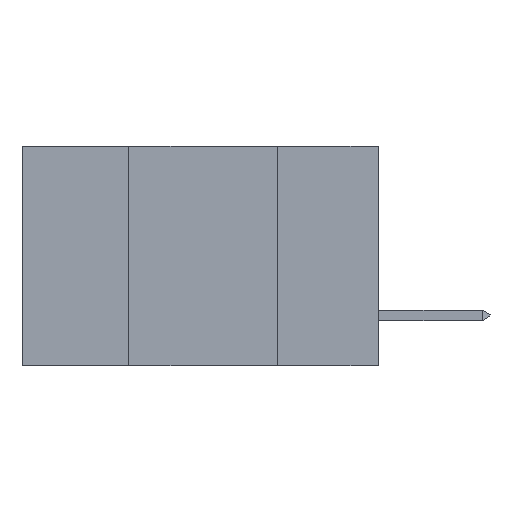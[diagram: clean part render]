
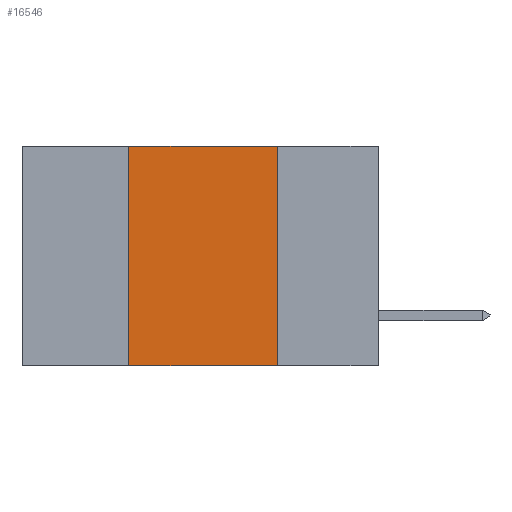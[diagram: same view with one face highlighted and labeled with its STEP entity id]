
A CAD part, left-side view. The second image highlights one B-rep face of the part: STEP entity #16546.
In plain terms, the highlighted planar face has unit normal (-1, 0, 0).
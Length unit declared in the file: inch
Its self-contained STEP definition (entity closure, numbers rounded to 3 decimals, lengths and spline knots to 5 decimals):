
#92 = CARTESIAN_POINT ( 'NONE',  ( 0., 0.42, -0.37 ) ) ;
#449 = DIRECTION ( 'NONE',  ( 0., -1., 0. ) ) ;
#776 = DIRECTION ( 'NONE',  ( 0., 0., -1. ) ) ;
#977 = CARTESIAN_POINT ( 'NONE',  ( 0., 0.17, -0.37 ) ) ;
#1224 = DIRECTION ( 'NONE',  ( 0., -1., 0. ) ) ;
#1528 = VERTEX_POINT ( 'NONE', #7493 ) ;
#1850 = VECTOR ( 'NONE', #1224, 39.37008 ) ;
#1912 = LINE ( 'NONE', #7753, #3052 ) ;
#3052 = VECTOR ( 'NONE', #449, 39.37008 ) ;
#4154 = DIRECTION ( 'NONE',  ( 0., 0., -1. ) ) ;
#5501 = PLANE ( 'NONE',  #15936 ) ;
#5685 = DIRECTION ( 'NONE',  ( 1., 0., 0. ) ) ;
#6849 = VERTEX_POINT ( 'NONE', #15124 ) ;
#6858 = EDGE_CURVE ( 'NONE', #6849, #8753, #1912, .T. ) ;
#7394 = ORIENTED_EDGE ( 'NONE', *, *, #6858, .T. ) ;
#7493 = CARTESIAN_POINT ( 'NONE',  ( 0., 0.17, 0. ) ) ;
#7753 = CARTESIAN_POINT ( 'NONE',  ( 0., 0.6, -0.37 ) ) ;
#8753 = VERTEX_POINT ( 'NONE', #17651 ) ;
#8805 = LINE ( 'NONE', #15787, #1850 ) ;
#9197 = EDGE_CURVE ( 'NONE', #6849, #15627, #12170, .T. ) ;
#9680 = ORIENTED_EDGE ( 'NONE', *, *, #15695, .F. ) ;
#9821 = LINE ( 'NONE', #977, #10634 ) ;
#10634 = VECTOR ( 'NONE', #776, 39.37008 ) ;
#11250 = VECTOR ( 'NONE', #17983, 39.37008 ) ;
#11438 = FACE_OUTER_BOUND ( 'NONE', #16389, .T. ) ;
#12170 = LINE ( 'NONE', #92, #11250 ) ;
#13056 = EDGE_CURVE ( 'NONE', #1528, #8753, #9821, .T. ) ;
#14536 = CARTESIAN_POINT ( 'NONE',  ( 0., 0.42, 0. ) ) ;
#15124 = CARTESIAN_POINT ( 'NONE',  ( 0., 0.42, -0.37 ) ) ;
#15508 = ORIENTED_EDGE ( 'NONE', *, *, #9197, .F. ) ;
#15627 = VERTEX_POINT ( 'NONE', #14536 ) ;
#15695 = EDGE_CURVE ( 'NONE', #15627, #1528, #8805, .T. ) ;
#15787 = CARTESIAN_POINT ( 'NONE',  ( 0., 0.6, 0. ) ) ;
#15936 = AXIS2_PLACEMENT_3D ( 'NONE', #17248, #5685, #4154 ) ;
#16389 = EDGE_LOOP ( 'NONE', ( #17124, #9680, #15508, #7394 ) ) ;
#16546 = ADVANCED_FACE ( 'NONE', ( #11438 ), #5501, .F. ) ;
#17124 = ORIENTED_EDGE ( 'NONE', *, *, #13056, .F. ) ;
#17248 = CARTESIAN_POINT ( 'NONE',  ( 0., 0.6, 0. ) ) ;
#17651 = CARTESIAN_POINT ( 'NONE',  ( 0., 0.17, -0.37 ) ) ;
#17983 = DIRECTION ( 'NONE',  ( 0., 0., 1. ) ) ;
